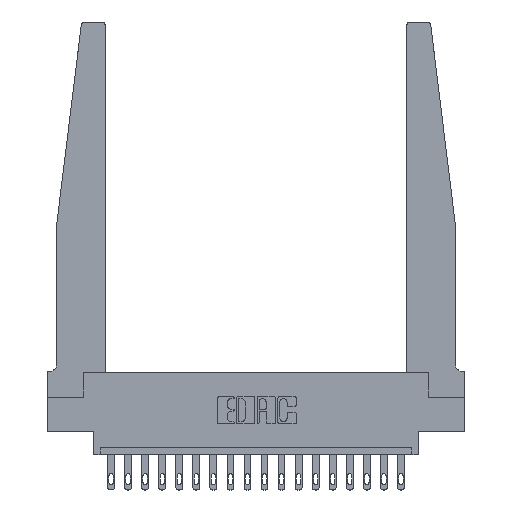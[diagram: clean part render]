
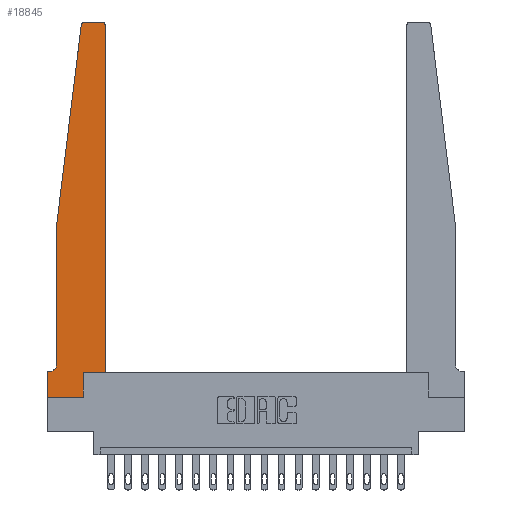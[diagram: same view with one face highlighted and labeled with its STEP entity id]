
A CAD part, top view. The second image highlights one B-rep face of the part: STEP entity #18845.
In plain terms, the highlighted planar face has unit normal (0, 0, 1).
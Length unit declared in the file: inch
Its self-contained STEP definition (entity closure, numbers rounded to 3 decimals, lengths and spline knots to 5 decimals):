
#19 = EDGE_CURVE ( 'NONE', #5612, #6718, #4511, .T. ) ;
#124 = CARTESIAN_POINT ( 'NONE',  ( 0.425, 0.18, 0.37 ) ) ;
#890 = EDGE_CURVE ( 'NONE', #19331, #1482, #17758, .T. ) ;
#1134 = CARTESIAN_POINT ( 'NONE',  ( 0.395, 2.75, 0.37 ) ) ;
#1482 = VERTEX_POINT ( 'NONE', #18494 ) ;
#1697 = EDGE_LOOP ( 'NONE', ( #4830, #16143, #4173, #16911, #18602, #17474, #13471, #8400, #15509, #8725, #3184, #7268 ) ) ;
#2462 = VERTEX_POINT ( 'NONE', #19609 ) ;
#2755 = VECTOR ( 'NONE', #11553, 39.37008 ) ;
#3184 = ORIENTED_EDGE ( 'NONE', *, *, #17291, .T. ) ;
#3467 = EDGE_CURVE ( 'NONE', #11188, #19506, #7581, .T. ) ;
#3471 = VECTOR ( 'NONE', #18275, 39.37008 ) ;
#3622 = CARTESIAN_POINT ( 'NONE',  ( 0.2605, 0.18, 0.37 ) ) ;
#4091 = DIRECTION ( 'NONE',  ( -1., 0., 0. ) ) ;
#4173 = ORIENTED_EDGE ( 'NONE', *, *, #10931, .T. ) ;
#4511 = LINE ( 'NONE', #12092, #7212 ) ;
#4543 = CARTESIAN_POINT ( 'NONE',  ( 0.27653, 2.75, 0.37 ) ) ;
#4546 = LINE ( 'NONE', #12228, #3471 ) ;
#4669 = VECTOR ( 'NONE', #4091, 39.37008 ) ;
#4830 = ORIENTED_EDGE ( 'NONE', *, *, #12753, .T. ) ;
#4872 = DIRECTION ( 'NONE',  ( -1., 0., 0. ) ) ;
#5088 = LINE ( 'NONE', #6764, #2755 ) ;
#5131 = AXIS2_PLACEMENT_3D ( 'NONE', #19296, #5679, #10462 ) ;
#5262 = AXIS2_PLACEMENT_3D ( 'NONE', #11098, #17143, #9602 ) ;
#5455 = VECTOR ( 'NONE', #9847, 39.37008 ) ;
#5612 = VERTEX_POINT ( 'NONE', #18718 ) ;
#5679 = DIRECTION ( 'NONE',  ( 0., 0., 1. ) ) ;
#5716 = EDGE_CURVE ( 'NONE', #9241, #13218, #17319, .T. ) ;
#5877 = CARTESIAN_POINT ( 'NONE',  ( 0.015, 0.1875, 0.37 ) ) ;
#6027 = VERTEX_POINT ( 'NONE', #9563 ) ;
#6084 = VECTOR ( 'NONE', #16152, 39.37008 ) ;
#6110 = DIRECTION ( 'NONE',  ( 1., 0., 0. ) ) ;
#6718 = VERTEX_POINT ( 'NONE', #13386 ) ;
#6764 = CARTESIAN_POINT ( 'NONE',  ( 0.065, 1.25, 0.37 ) ) ;
#6788 = DIRECTION ( 'NONE',  ( 0., 0., 1. ) ) ;
#7153 = FACE_OUTER_BOUND ( 'NONE', #1697, .T. ) ;
#7212 = VECTOR ( 'NONE', #6110, 39.37008 ) ;
#7268 = ORIENTED_EDGE ( 'NONE', *, *, #3467, .T. ) ;
#7581 = CIRCLE ( 'NONE', #9506, 0.03 ) ;
#8240 = AXIS2_PLACEMENT_3D ( 'NONE', #13819, #12141, #16901 ) ;
#8300 = EDGE_CURVE ( 'NONE', #13218, #5612, #8899, .T. ) ;
#8400 = ORIENTED_EDGE ( 'NONE', *, *, #19, .T. ) ;
#8508 = VERTEX_POINT ( 'NONE', #3622 ) ;
#8665 = DIRECTION ( 'NONE',  ( -0.122, -0.992, 0. ) ) ;
#8725 = ORIENTED_EDGE ( 'NONE', *, *, #18980, .T. ) ;
#8899 = LINE ( 'NONE', #16350, #12248 ) ;
#8917 = EDGE_CURVE ( 'NONE', #2462, #9241, #13851, .T. ) ;
#9241 = VERTEX_POINT ( 'NONE', #5877 ) ;
#9396 = EDGE_CURVE ( 'NONE', #6027, #2462, #5088, .T. ) ;
#9506 = AXIS2_PLACEMENT_3D ( 'NONE', #12963, #6788, #17530 ) ;
#9563 = CARTESIAN_POINT ( 'NONE',  ( 0.065, 1.25, 0.37 ) ) ;
#9602 = DIRECTION ( 'NONE',  ( -1., 0., 0. ) ) ;
#9847 = DIRECTION ( 'NONE',  ( 1., 0., 0. ) ) ;
#10105 = VECTOR ( 'NONE', #4872, 39.37008 ) ;
#10263 = CARTESIAN_POINT ( 'NONE',  ( 0.065, 1.25, 0.37 ) ) ;
#10462 = DIRECTION ( 'NONE',  ( 1., 0., 0. ) ) ;
#10931 = EDGE_CURVE ( 'NONE', #1482, #6027, #16616, .T. ) ;
#10951 = LINE ( 'NONE', #14035, #10105 ) ;
#11098 = CARTESIAN_POINT ( 'NONE',  ( 0.015, 0.2375, 0.37 ) ) ;
#11188 = VERTEX_POINT ( 'NONE', #14797 ) ;
#11553 = DIRECTION ( 'NONE',  ( 0., -1., 0. ) ) ;
#12092 = CARTESIAN_POINT ( 'NONE',  ( 0., 0., 0.37 ) ) ;
#12141 = DIRECTION ( 'NONE',  ( 0., 0., 1. ) ) ;
#12228 = CARTESIAN_POINT ( 'NONE',  ( 0.2605, 0.18, 0.37 ) ) ;
#12248 = VECTOR ( 'NONE', #14665, 39.37008 ) ;
#12753 = EDGE_CURVE ( 'NONE', #19506, #19331, #10951, .T. ) ;
#12758 = CARTESIAN_POINT ( 'NONE',  ( 0.065, 0.1875, 0.37 ) ) ;
#12963 = CARTESIAN_POINT ( 'NONE',  ( 0.395, 2.72, 0.37 ) ) ;
#13218 = VERTEX_POINT ( 'NONE', #15892 ) ;
#13236 = PLANE ( 'NONE',  #5131 ) ;
#13386 = CARTESIAN_POINT ( 'NONE',  ( 0.2605, 0., 0.37 ) ) ;
#13457 = LINE ( 'NONE', #19519, #6084 ) ;
#13471 = ORIENTED_EDGE ( 'NONE', *, *, #8300, .T. ) ;
#13819 = CARTESIAN_POINT ( 'NONE',  ( 0.27653, 2.72, 0.37 ) ) ;
#13851 = CIRCLE ( 'NONE', #5262, 0.05 ) ;
#14035 = CARTESIAN_POINT ( 'NONE',  ( 0.25, 2.75, 0.37 ) ) ;
#14305 = EDGE_CURVE ( 'NONE', #6718, #8508, #4546, .T. ) ;
#14665 = DIRECTION ( 'NONE',  ( 0., -1., 0. ) ) ;
#14797 = CARTESIAN_POINT ( 'NONE',  ( 0.425, 2.72, 0.37 ) ) ;
#15509 = ORIENTED_EDGE ( 'NONE', *, *, #14305, .T. ) ;
#15892 = CARTESIAN_POINT ( 'NONE',  ( 0., 0.1875, 0.37 ) ) ;
#16143 = ORIENTED_EDGE ( 'NONE', *, *, #890, .T. ) ;
#16152 = DIRECTION ( 'NONE',  ( 0., 1., 0. ) ) ;
#16350 = CARTESIAN_POINT ( 'NONE',  ( 0., 0., 0.37 ) ) ;
#16616 = LINE ( 'NONE', #10263, #18981 ) ;
#16901 = DIRECTION ( 'NONE',  ( 1., 0., 0. ) ) ;
#16911 = ORIENTED_EDGE ( 'NONE', *, *, #9396, .T. ) ;
#17143 = DIRECTION ( 'NONE',  ( 0., 0., -1. ) ) ;
#17291 = EDGE_CURVE ( 'NONE', #18503, #11188, #13457, .T. ) ;
#17299 = LINE ( 'NONE', #17485, #5455 ) ;
#17319 = LINE ( 'NONE', #12758, #4669 ) ;
#17474 = ORIENTED_EDGE ( 'NONE', *, *, #5716, .T. ) ;
#17485 = CARTESIAN_POINT ( 'NONE',  ( 0.425, 0.18, 0.37 ) ) ;
#17530 = DIRECTION ( 'NONE',  ( 1., 0., 0. ) ) ;
#17758 = CIRCLE ( 'NONE', #8240, 0.03 ) ;
#18275 = DIRECTION ( 'NONE',  ( 0., 1., 0. ) ) ;
#18494 = CARTESIAN_POINT ( 'NONE',  ( 0.24675, 2.72367, 0.37 ) ) ;
#18503 = VERTEX_POINT ( 'NONE', #124 ) ;
#18602 = ORIENTED_EDGE ( 'NONE', *, *, #8917, .T. ) ;
#18718 = CARTESIAN_POINT ( 'NONE',  ( 0., 0., 0.37 ) ) ;
#18845 = ADVANCED_FACE ( 'NONE', ( #7153 ), #13236, .T. ) ;
#18980 = EDGE_CURVE ( 'NONE', #8508, #18503, #17299, .T. ) ;
#18981 = VECTOR ( 'NONE', #8665, 39.37008 ) ;
#19296 = CARTESIAN_POINT ( 'NONE',  ( 0., 0.1875, 0.37 ) ) ;
#19331 = VERTEX_POINT ( 'NONE', #4543 ) ;
#19506 = VERTEX_POINT ( 'NONE', #1134 ) ;
#19519 = CARTESIAN_POINT ( 'NONE',  ( 0.425, 0.18, 0.37 ) ) ;
#19609 = CARTESIAN_POINT ( 'NONE',  ( 0.065, 0.2375, 0.37 ) ) ;
